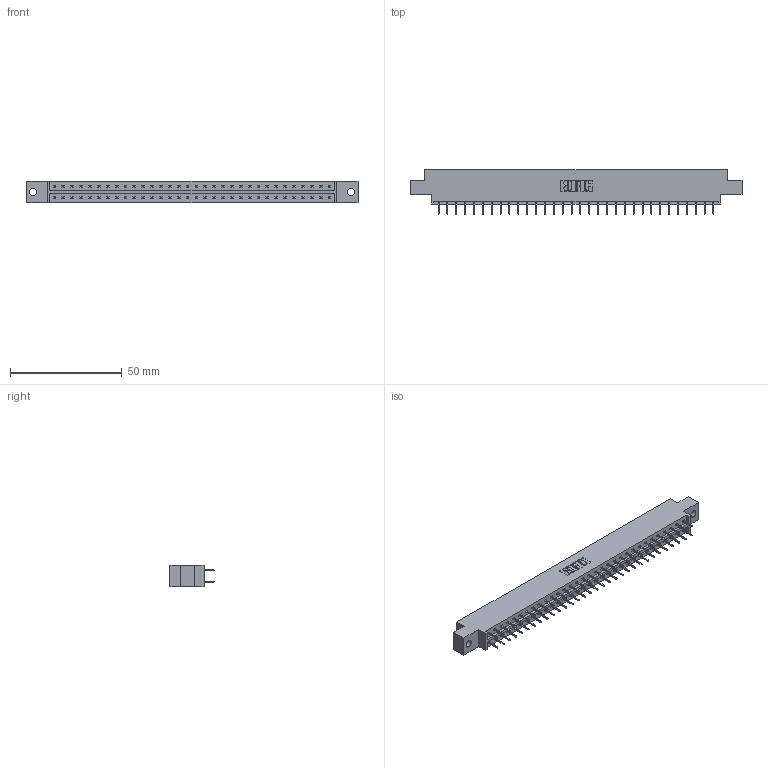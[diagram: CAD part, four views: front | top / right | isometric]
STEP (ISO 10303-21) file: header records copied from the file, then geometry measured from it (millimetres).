
FILE_DESCRIPTION (( 'STEP AP203' ), '1' );
FILE_NAME ('833-064-524-802.STEP', '2020-06-05T07:05:40', ( '' ), ( '' ), 'SwSTEP 2.0', 'SolidWorks 2020', '' );
FILE_SCHEMA (( 'CONFIG_CONTROL_DESIGN' ));
Length unit declared in the file: inch
Products named in the file (3): 833 Part_Offset - .128 Dia; 833-064-524-802; 345-292-001_345-293-124
Assembly tree (65 placements, depth 2):
  833-064-524-802
    833 Part_Offset - .128 Dia
    345-292-001_345-293-124  x64
Bounding box: 148.34 x 19.69 x 9.4 mm (x, y, z)
Volume: 14689.4 mm3; surface area: 16915.9 mm2
Topology: 65 solids, 65 shells, 3702 faces, 10499 edges, 6742 vertices
Faces by surface type: plane 2762, cylinder 940
Entity records: 22089 total; most frequent: CARTESIAN_POINT 3674, ORIENTED_EDGE 3610, DIRECTION 3157, EDGE_CURVE 1805, LINE 1681, VECTOR 1681, VERTEX_POINT 1198, AXIS2_PLACEMENT_3D 738
